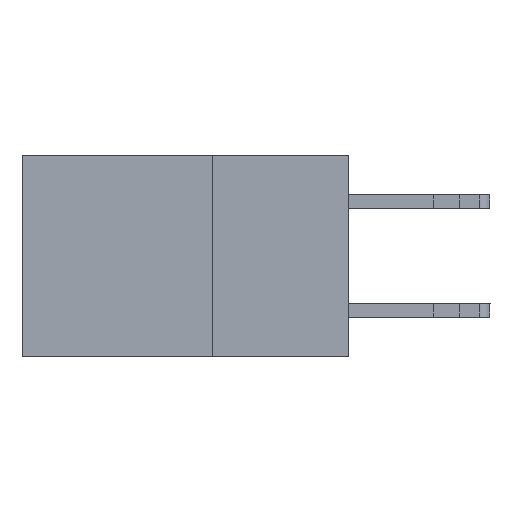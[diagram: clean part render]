
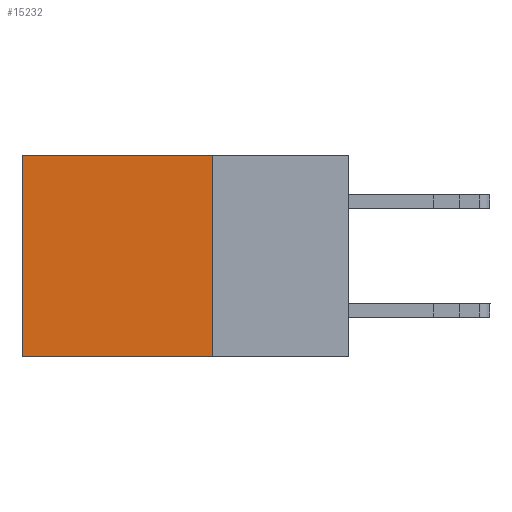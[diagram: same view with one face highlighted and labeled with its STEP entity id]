
A CAD part, left-side view. The second image highlights one B-rep face of the part: STEP entity #15232.
In plain terms, the highlighted planar face has unit normal (-1, 0, 0).
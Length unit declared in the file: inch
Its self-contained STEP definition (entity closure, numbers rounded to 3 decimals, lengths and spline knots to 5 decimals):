
#173 = PLANE ( 'NONE',  #5048 ) ;
#1097 = CARTESIAN_POINT ( 'NONE',  ( 0.2615, 0.25, 0. ) ) ;
#1386 = DIRECTION ( 'NONE',  ( 0., 1., 0. ) ) ;
#1904 = VECTOR ( 'NONE', #7826, 39.37008 ) ;
#2202 = CARTESIAN_POINT ( 'NONE',  ( 0.2615, 0.6, -0.37 ) ) ;
#3066 = DIRECTION ( 'NONE',  ( 1., 0., 0. ) ) ;
#4297 = FACE_OUTER_BOUND ( 'NONE', #10022, .T. ) ;
#4354 = VERTEX_POINT ( 'NONE', #4709 ) ;
#4709 = CARTESIAN_POINT ( 'NONE',  ( 0.2615, 0.6, 0. ) ) ;
#4829 = EDGE_CURVE ( 'NONE', #12167, #4354, #14092, .T. ) ;
#5048 = AXIS2_PLACEMENT_3D ( 'NONE', #11340, #3066, #12751 ) ;
#5065 = ORIENTED_EDGE ( 'NONE', *, *, #4829, .T. ) ;
#5263 = ORIENTED_EDGE ( 'NONE', *, *, #17583, .F. ) ;
#6087 = VECTOR ( 'NONE', #11638, 39.37008 ) ;
#6286 = VECTOR ( 'NONE', #13431, 39.37008 ) ;
#6452 = VECTOR ( 'NONE', #1386, 39.37008 ) ;
#6934 = ORIENTED_EDGE ( 'NONE', *, *, #15119, .F. ) ;
#7301 = VERTEX_POINT ( 'NONE', #2202 ) ;
#7645 = CARTESIAN_POINT ( 'NONE',  ( 0.2615, 0.25, -0.37 ) ) ;
#7826 = DIRECTION ( 'NONE',  ( 0., 0., -1. ) ) ;
#8709 = VERTEX_POINT ( 'NONE', #7645 ) ;
#10022 = EDGE_LOOP ( 'NONE', ( #12393, #6934, #5263, #5065 ) ) ;
#10658 = LINE ( 'NONE', #14417, #6087 ) ;
#11095 = CARTESIAN_POINT ( 'NONE',  ( 0.2615, 0.25, -0.37 ) ) ;
#11340 = CARTESIAN_POINT ( 'NONE',  ( 0.2615, 0.25, -0.37 ) ) ;
#11638 = DIRECTION ( 'NONE',  ( 0., 0., -1. ) ) ;
#12167 = VERTEX_POINT ( 'NONE', #1097 ) ;
#12393 = ORIENTED_EDGE ( 'NONE', *, *, #12591, .T. ) ;
#12591 = EDGE_CURVE ( 'NONE', #4354, #7301, #10658, .T. ) ;
#12751 = DIRECTION ( 'NONE',  ( 0., 0., -1. ) ) ;
#13431 = DIRECTION ( 'NONE',  ( 0., 1., 0. ) ) ;
#14092 = LINE ( 'NONE', #14811, #6286 ) ;
#14417 = CARTESIAN_POINT ( 'NONE',  ( 0.2615, 0.6, -0.37 ) ) ;
#14811 = CARTESIAN_POINT ( 'NONE',  ( 0.2615, 0.25, 0. ) ) ;
#15119 = EDGE_CURVE ( 'NONE', #8709, #7301, #16989, .T. ) ;
#15232 = ADVANCED_FACE ( 'NONE', ( #4297 ), #173, .F. ) ;
#16088 = CARTESIAN_POINT ( 'NONE',  ( 0.2615, 0.25, -0.37 ) ) ;
#16184 = LINE ( 'NONE', #16088, #1904 ) ;
#16989 = LINE ( 'NONE', #11095, #6452 ) ;
#17583 = EDGE_CURVE ( 'NONE', #12167, #8709, #16184, .T. ) ;
